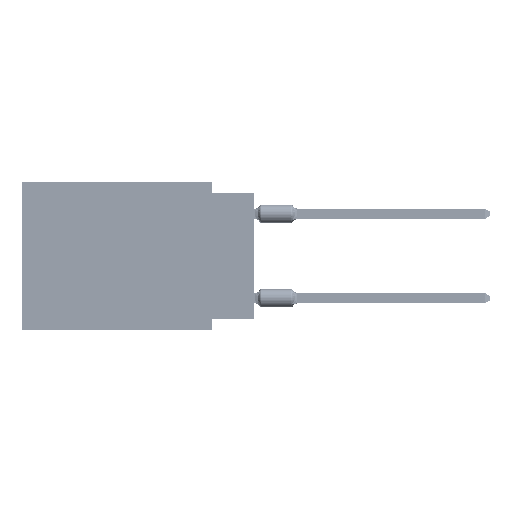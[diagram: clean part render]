
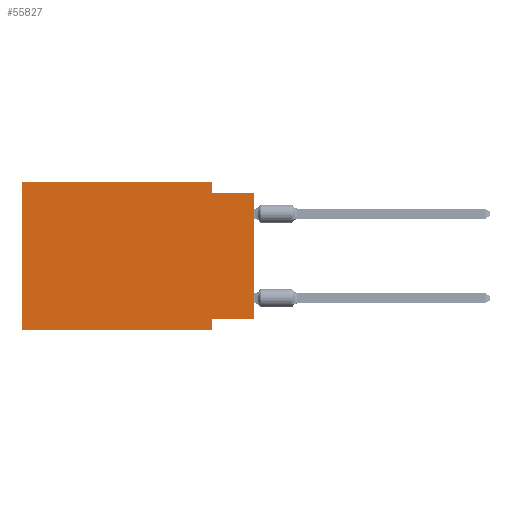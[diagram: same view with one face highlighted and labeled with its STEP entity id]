
A CAD part, left-side view. The second image highlights one B-rep face of the part: STEP entity #55827.
In plain terms, the highlighted planar face has unit normal (-1, 0, 0).
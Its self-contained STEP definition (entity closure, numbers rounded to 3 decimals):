
#28 = VECTOR ( 'NONE', #63794, 1000. ) ;
#143 = DIRECTION ( 'NONE',  ( 0., -1., 0. ) ) ;
#470 = EDGE_CURVE ( 'NONE', #62463, #53282, #34850, .T. ) ;
#789 = CARTESIAN_POINT ( 'NONE',  ( 0., 0., 0. ) ) ;
#1389 = VERTEX_POINT ( 'NONE', #49504 ) ;
#1682 = LINE ( 'NONE', #8622, #28 ) ;
#2339 = EDGE_LOOP ( 'NONE', ( #68554, #41615, #49667, #62266, #5021, #28106, #56645, #32364 ) ) ;
#2959 = CARTESIAN_POINT ( 'NONE',  ( 0., 13.97, 0. ) ) ;
#3817 = CARTESIAN_POINT ( 'NONE',  ( 0., 2.54, -8.89 ) ) ;
#3928 = EDGE_CURVE ( 'NONE', #54550, #7976, #1682, .T. ) ;
#4140 = VECTOR ( 'NONE', #143, 1000. ) ;
#5021 = ORIENTED_EDGE ( 'NONE', *, *, #470, .F. ) ;
#6118 = LINE ( 'NONE', #60238, #13314 ) ;
#6906 = CARTESIAN_POINT ( 'NONE',  ( 0., 2.54, 0. ) ) ;
#7793 = DIRECTION ( 'NONE',  ( 0., 0., 1. ) ) ;
#7976 = VERTEX_POINT ( 'NONE', #54433 ) ;
#8622 = CARTESIAN_POINT ( 'NONE',  ( 0., 0., -8.255 ) ) ;
#10402 = LINE ( 'NONE', #22062, #4140 ) ;
#12004 = AXIS2_PLACEMENT_3D ( 'NONE', #2959, #47540, #65064 ) ;
#12833 = DIRECTION ( 'NONE',  ( 0., 0., 1. ) ) ;
#12927 = VECTOR ( 'NONE', #33626, 1000. ) ;
#13314 = VECTOR ( 'NONE', #22920, 1000. ) ;
#13575 = CARTESIAN_POINT ( 'NONE',  ( 0., 13.97, 0. ) ) ;
#14430 = LINE ( 'NONE', #3817, #39320 ) ;
#15119 = CARTESIAN_POINT ( 'NONE',  ( 0., 13.97, 0. ) ) ;
#16829 = CARTESIAN_POINT ( 'NONE',  ( 0., 0., -8.255 ) ) ;
#19507 = CARTESIAN_POINT ( 'NONE',  ( 0., 0., -0.635 ) ) ;
#19513 = DIRECTION ( 'NONE',  ( 0., -1., 0. ) ) ;
#19623 = VERTEX_POINT ( 'NONE', #22411 ) ;
#19773 = PLANE ( 'NONE',  #12004 ) ;
#22062 = CARTESIAN_POINT ( 'NONE',  ( 0., 0., -0.635 ) ) ;
#22411 = CARTESIAN_POINT ( 'NONE',  ( 0., 2.54, 0. ) ) ;
#22920 = DIRECTION ( 'NONE',  ( 0., -1., 0. ) ) ;
#25011 = DIRECTION ( 'NONE',  ( 0., 0., -1. ) ) ;
#26676 = CARTESIAN_POINT ( 'NONE',  ( 0., 13.97, -8.89 ) ) ;
#28106 = ORIENTED_EDGE ( 'NONE', *, *, #58869, .T. ) ;
#29350 = CARTESIAN_POINT ( 'NONE',  ( 0., 13.97, 0. ) ) ;
#30043 = VECTOR ( 'NONE', #7793, 1000. ) ;
#32364 = ORIENTED_EDGE ( 'NONE', *, *, #3928, .F. ) ;
#33365 = VECTOR ( 'NONE', #12833, 1000. ) ;
#33626 = DIRECTION ( 'NONE',  ( 0., 0., -1. ) ) ;
#33965 = VERTEX_POINT ( 'NONE', #19507 ) ;
#34184 = EDGE_CURVE ( 'NONE', #54550, #33965, #68730, .T. ) ;
#34850 = LINE ( 'NONE', #29350, #30043 ) ;
#39320 = VECTOR ( 'NONE', #25011, 1000. ) ;
#41615 = ORIENTED_EDGE ( 'NONE', *, *, #47267, .F. ) ;
#42311 = EDGE_CURVE ( 'NONE', #19623, #1389, #62449, .T. ) ;
#45222 = VERTEX_POINT ( 'NONE', #51473 ) ;
#46600 = VECTOR ( 'NONE', #19513, 1000. ) ;
#47267 = EDGE_CURVE ( 'NONE', #1389, #33965, #10402, .T. ) ;
#47540 = DIRECTION ( 'NONE',  ( 1., 0., 0. ) ) ;
#49504 = CARTESIAN_POINT ( 'NONE',  ( 0., 2.54, -0.635 ) ) ;
#49667 = ORIENTED_EDGE ( 'NONE', *, *, #42311, .F. ) ;
#50333 = EDGE_CURVE ( 'NONE', #7976, #45222, #14430, .T. ) ;
#51473 = CARTESIAN_POINT ( 'NONE',  ( 0., 2.54, -8.89 ) ) ;
#52836 = EDGE_CURVE ( 'NONE', #53282, #19623, #69541, .T. ) ;
#53282 = VERTEX_POINT ( 'NONE', #13575 ) ;
#54433 = CARTESIAN_POINT ( 'NONE',  ( 0., 2.54, -8.255 ) ) ;
#54550 = VERTEX_POINT ( 'NONE', #16829 ) ;
#55827 = ADVANCED_FACE ( 'NONE', ( #64703 ), #19773, .F. ) ;
#56645 = ORIENTED_EDGE ( 'NONE', *, *, #50333, .F. ) ;
#58869 = EDGE_CURVE ( 'NONE', #62463, #45222, #6118, .T. ) ;
#60238 = CARTESIAN_POINT ( 'NONE',  ( 0., 13.97, -8.89 ) ) ;
#62266 = ORIENTED_EDGE ( 'NONE', *, *, #52836, .F. ) ;
#62449 = LINE ( 'NONE', #6906, #12927 ) ;
#62463 = VERTEX_POINT ( 'NONE', #26676 ) ;
#63794 = DIRECTION ( 'NONE',  ( 0., 1., 0. ) ) ;
#64703 = FACE_OUTER_BOUND ( 'NONE', #2339, .T. ) ;
#65064 = DIRECTION ( 'NONE',  ( 0., 0., -1. ) ) ;
#68554 = ORIENTED_EDGE ( 'NONE', *, *, #34184, .T. ) ;
#68730 = LINE ( 'NONE', #789, #33365 ) ;
#69541 = LINE ( 'NONE', #15119, #46600 ) ;
